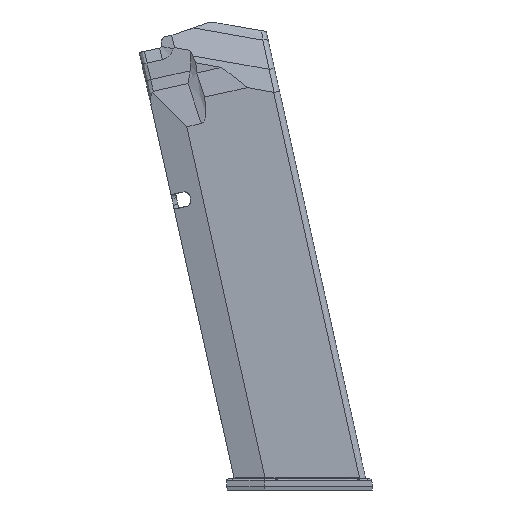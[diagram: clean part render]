
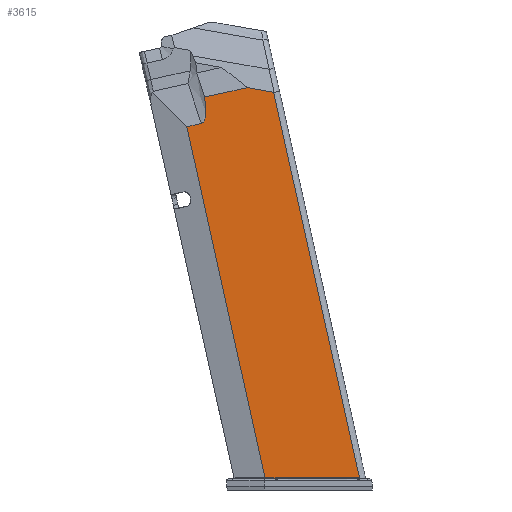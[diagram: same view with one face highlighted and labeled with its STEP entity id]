
A CAD part, left-side view. The second image highlights one B-rep face of the part: STEP entity #3615.
In plain terms, the highlighted planar face has unit normal (-1, 0, 0).
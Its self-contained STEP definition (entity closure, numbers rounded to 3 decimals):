
#116=B_SPLINE_CURVE_WITH_KNOTS('',3,(#5649,#5650,#5651,#5652,#5653,#5654,
#5655,#5656,#5657,#5658,#5659,#5660,#5661),.UNSPECIFIED.,.F.,.F.,(4,3,3,
3,4),(0.433,0.612,0.907,1.091,
1.202),.UNSPECIFIED.);
#354=FACE_OUTER_BOUND('',#560,.T.);
#560=EDGE_LOOP('',(#2586,#2587,#2588,#2589,#2590,#2591,#2592,#2593));
#745=ELLIPSE('',#3836,1.083,0.25);
#880=LINE('',#5249,#1159);
#886=LINE('',#5272,#1165);
#942=LINE('',#5616,#1221);
#945=LINE('',#5663,#1224);
#946=LINE('',#5664,#1225);
#947=LINE('',#5665,#1226);
#1159=VECTOR('',#4074,10.);
#1165=VECTOR('',#4086,10.039);
#1221=VECTOR('',#4210,10.04);
#1224=VECTOR('',#4223,10.038);
#1225=VECTOR('',#4224,10.002);
#1226=VECTOR('',#4225,10.002);
#1456=VERTEX_POINT('',#5234);
#1457=VERTEX_POINT('',#5248);
#1463=VERTEX_POINT('',#5271);
#1516=VERTEX_POINT('',#5527);
#1517=VERTEX_POINT('',#5529);
#1523=VERTEX_POINT('',#5607);
#1528=VERTEX_POINT('',#5648);
#1529=VERTEX_POINT('',#5662);
#1834=EDGE_CURVE('',#1457,#1456,#880,.T.);
#1842=EDGE_CURVE('',#1457,#1463,#886,.T.);
#1916=EDGE_CURVE('',#1516,#1517,#745,.T.);
#1928=EDGE_CURVE('',#1523,#1516,#942,.T.);
#1935=EDGE_CURVE('',#1528,#1456,#116,.F.);
#1936=EDGE_CURVE('',#1529,#1528,#945,.T.);
#1937=EDGE_CURVE('',#1529,#1517,#946,.T.);
#1938=EDGE_CURVE('',#1463,#1523,#947,.T.);
#2586=ORIENTED_EDGE('',*,*,#1834,.T.);
#2587=ORIENTED_EDGE('',*,*,#1935,.F.);
#2588=ORIENTED_EDGE('',*,*,#1936,.F.);
#2589=ORIENTED_EDGE('',*,*,#1937,.T.);
#2590=ORIENTED_EDGE('',*,*,#1916,.F.);
#2591=ORIENTED_EDGE('',*,*,#1928,.F.);
#2592=ORIENTED_EDGE('',*,*,#1938,.F.);
#2593=ORIENTED_EDGE('',*,*,#1842,.F.);
#3510=PLANE('',#3849);
#3615=ADVANCED_FACE('',(#354),#3510,.T.);
#3836=AXIS2_PLACEMENT_3D('',#5530,#4189,#4190);
#3849=AXIS2_PLACEMENT_3D('',#5647,#4221,#4222);
#4074=DIRECTION('',(0.,0.976,-0.217));
#4086=DIRECTION('',(0.,-0.985,-0.173));
#4189=DIRECTION('center_axis',(-1.,0.,0.));
#4190=DIRECTION('ref_axis',(0.,-1.,0.));
#4210=DIRECTION('',(0.,1.,0.));
#4221=DIRECTION('center_axis',(-1.,0.,0.));
#4222=DIRECTION('ref_axis',(0.,0.,1.));
#4223=DIRECTION('',(0.,-0.976,0.216));
#4224=DIRECTION('',(0.,-0.217,-0.976));
#4225=DIRECTION('',(0.,-0.217,-0.976));
#5234=CARTESIAN_POINT('',(-10.542,24.794,99.857));
#5248=CARTESIAN_POINT('',(-10.542,14.048,102.249));
#5249=CARTESIAN_POINT('',(-10.542,15.441,101.939));
#5271=CARTESIAN_POINT('',(-10.542,7.312,101.067));
#5272=CARTESIAN_POINT('',(-10.542,-11.626,97.741));
#5527=CARTESIAN_POINT('',(-10.542,9.51,3.05));
#5529=CARTESIAN_POINT('',(-10.542,9.511,3.063));
#5530=CARTESIAN_POINT('Origin',(-10.542,10.592,3.05));
#5607=CARTESIAN_POINT('',(-10.542,-14.504,3.05));
#5616=CARTESIAN_POINT('',(-10.542,-9.248,3.05));
#5647=CARTESIAN_POINT('Origin',(-10.542,-19.459,-12.279));
#5648=CARTESIAN_POINT('',(-10.542,25.666,93.142));
#5649=CARTESIAN_POINT('Ctrl Pts',(-10.542,24.794,99.857));
#5650=CARTESIAN_POINT('Ctrl Pts',(-10.542,24.726,99.253));
#5651=CARTESIAN_POINT('Ctrl Pts',(-10.542,24.668,98.644));
#5652=CARTESIAN_POINT('Ctrl Pts',(-10.542,24.628,98.003));
#5653=CARTESIAN_POINT('Ctrl Pts',(-10.542,24.561,96.95));
#5654=CARTESIAN_POINT('Ctrl Pts',(-10.542,24.549,95.875));
#5655=CARTESIAN_POINT('Ctrl Pts',(-10.542,24.665,95.003));
#5656=CARTESIAN_POINT('Ctrl Pts',(-10.542,24.737,94.458));
#5657=CARTESIAN_POINT('Ctrl Pts',(-10.542,24.846,93.987));
#5658=CARTESIAN_POINT('Ctrl Pts',(-10.542,25.076,93.611));
#5659=CARTESIAN_POINT('Ctrl Pts',(-10.542,25.215,93.384));
#5660=CARTESIAN_POINT('Ctrl Pts',(-10.542,25.413,93.198));
#5661=CARTESIAN_POINT('Ctrl Pts',(-10.542,25.666,93.142));
#5662=CARTESIAN_POINT('',(-10.542,29.379,92.322));
#5663=CARTESIAN_POINT('',(-10.542,20.949,94.184));
#5664=CARTESIAN_POINT('',(-10.542,4.899,-17.657));
#5665=CARTESIAN_POINT('',(-10.542,-17.989,-12.603));
